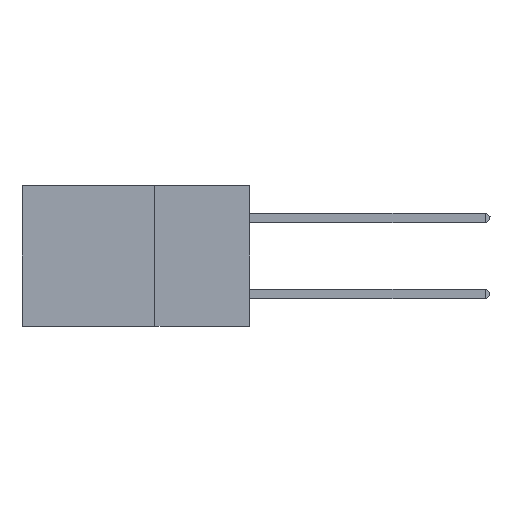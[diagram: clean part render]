
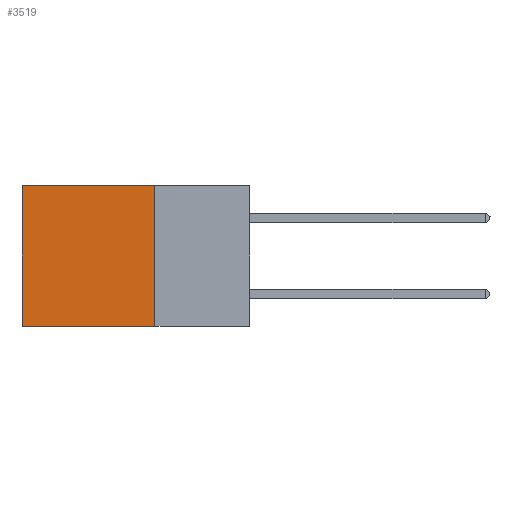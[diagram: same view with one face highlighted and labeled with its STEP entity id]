
A CAD part, left-side view. The second image highlights one B-rep face of the part: STEP entity #3519.
In plain terms, the highlighted planar face has unit normal (-1, 0, 0).
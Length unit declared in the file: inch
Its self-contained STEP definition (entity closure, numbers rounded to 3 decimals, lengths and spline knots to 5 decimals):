
#314 = PLANE ( 'NONE',  #9084 ) ;
#2095 = DIRECTION ( 'NONE',  ( 1., 0., 0. ) ) ;
#2327 = VECTOR ( 'NONE', #17079, 39.37008 ) ;
#2538 = VERTEX_POINT ( 'NONE', #7843 ) ;
#3519 = ADVANCED_FACE ( 'NONE', ( #18633 ), #314, .F. ) ;
#3599 = VERTEX_POINT ( 'NONE', #7596 ) ;
#5672 = CARTESIAN_POINT ( 'NONE',  ( 0.2875, 0.25, 0. ) ) ;
#6973 = ORIENTED_EDGE ( 'NONE', *, *, #20472, .T. ) ;
#6990 = DIRECTION ( 'NONE',  ( 0., 0., -1. ) ) ;
#7596 = CARTESIAN_POINT ( 'NONE',  ( 0.2875, 0.25, 0. ) ) ;
#7743 = ORIENTED_EDGE ( 'NONE', *, *, #17115, .F. ) ;
#7843 = CARTESIAN_POINT ( 'NONE',  ( 0.2875, 0.6, 0. ) ) ;
#8114 = EDGE_CURVE ( 'NONE', #3599, #2538, #10429, .T. ) ;
#8214 = DIRECTION ( 'NONE',  ( 0., 1., 0. ) ) ;
#9015 = EDGE_CURVE ( 'NONE', #11210, #10419, #9434, .T. ) ;
#9049 = LINE ( 'NONE', #5672, #2327 ) ;
#9084 = AXIS2_PLACEMENT_3D ( 'NONE', #18089, #2095, #6990 ) ;
#9278 = EDGE_LOOP ( 'NONE', ( #6973, #19009, #7743, #12648 ) ) ;
#9434 = LINE ( 'NONE', #19426, #13924 ) ;
#9492 = DIRECTION ( 'NONE',  ( 0., 1., 0. ) ) ;
#9942 = VECTOR ( 'NONE', #11934, 39.37008 ) ;
#10419 = VERTEX_POINT ( 'NONE', #20301 ) ;
#10429 = LINE ( 'NONE', #15872, #15210 ) ;
#11210 = VERTEX_POINT ( 'NONE', #12008 ) ;
#11851 = CARTESIAN_POINT ( 'NONE',  ( 0.2875, 0.6, 0. ) ) ;
#11934 = DIRECTION ( 'NONE',  ( 0., 0., -1. ) ) ;
#12008 = CARTESIAN_POINT ( 'NONE',  ( 0.2875, 0.25, -0.37 ) ) ;
#12648 = ORIENTED_EDGE ( 'NONE', *, *, #8114, .T. ) ;
#13924 = VECTOR ( 'NONE', #8214, 39.37008 ) ;
#15210 = VECTOR ( 'NONE', #9492, 39.37008 ) ;
#15872 = CARTESIAN_POINT ( 'NONE',  ( 0.2875, 0.25, 0. ) ) ;
#17079 = DIRECTION ( 'NONE',  ( 0., 0., -1. ) ) ;
#17115 = EDGE_CURVE ( 'NONE', #3599, #11210, #9049, .T. ) ;
#18089 = CARTESIAN_POINT ( 'NONE',  ( 0.2875, 0.25, 0. ) ) ;
#18633 = FACE_OUTER_BOUND ( 'NONE', #9278, .T. ) ;
#19009 = ORIENTED_EDGE ( 'NONE', *, *, #9015, .F. ) ;
#19398 = LINE ( 'NONE', #11851, #9942 ) ;
#19426 = CARTESIAN_POINT ( 'NONE',  ( 0.2875, 0.25, -0.37 ) ) ;
#20301 = CARTESIAN_POINT ( 'NONE',  ( 0.2875, 0.6, -0.37 ) ) ;
#20472 = EDGE_CURVE ( 'NONE', #2538, #10419, #19398, .T. ) ;
